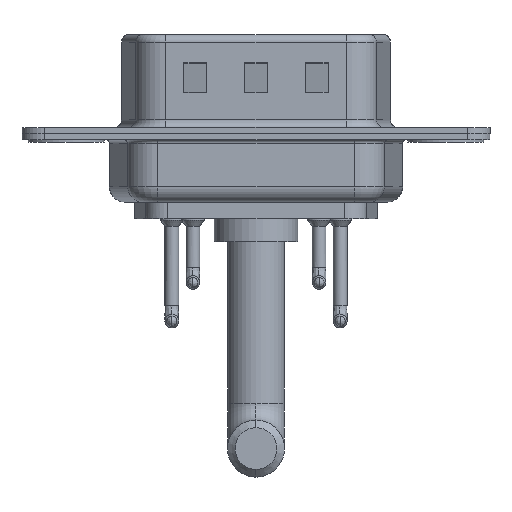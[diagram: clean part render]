
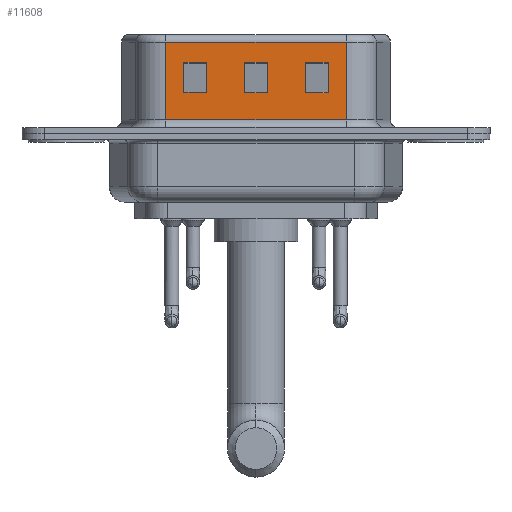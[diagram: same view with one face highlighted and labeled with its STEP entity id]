
A CAD part, front view. The second image highlights one B-rep face of the part: STEP entity #11608.
In plain terms, the highlighted planar face has unit normal (0, -1, 0).
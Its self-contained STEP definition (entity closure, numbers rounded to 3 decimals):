
#83 = ORIENTED_EDGE ( 'NONE', *, *, #14806, .T. ) ;
#181 = FACE_BOUND ( 'NONE', #15882, .T. ) ;
#237 = VECTOR ( 'NONE', #14333, 1000. ) ;
#532 = FACE_BOUND ( 'NONE', #3598, .T. ) ;
#615 = VERTEX_POINT ( 'NONE', #9459 ) ;
#1077 = CARTESIAN_POINT ( 'NONE',  ( 13.25, -4.55, 6.52 ) ) ;
#1397 = VERTEX_POINT ( 'NONE', #10139 ) ;
#1428 = AXIS2_PLACEMENT_3D ( 'NONE', #8686, #1691, #15089 ) ;
#1483 = CARTESIAN_POINT ( 'NONE',  ( 14.451, -4.55, 2.705 ) ) ;
#1499 = VERTEX_POINT ( 'NONE', #5333 ) ;
#1521 = VECTOR ( 'NONE', #3390, 1000. ) ;
#1559 = EDGE_CURVE ( 'NONE', #11625, #6355, #14482, .T. ) ;
#1678 = LINE ( 'NONE', #13912, #11077 ) ;
#1691 = DIRECTION ( 'NONE',  ( 0., 1., 0. ) ) ;
#1824 = CARTESIAN_POINT ( 'NONE',  ( 18.451, -4.55, 4.705 ) ) ;
#1938 = ORIENTED_EDGE ( 'NONE', *, *, #15453, .T. ) ;
#1942 = DIRECTION ( 'NONE',  ( -1., 0., 0. ) ) ;
#1975 = CARTESIAN_POINT ( 'NONE',  ( 6.549, -4.55, 6.52 ) ) ;
#2081 = VECTOR ( 'NONE', #13162, 1000. ) ;
#2189 = EDGE_CURVE ( 'NONE', #9253, #6253, #11804, .T. ) ;
#2249 = VECTOR ( 'NONE', #6692, 1000. ) ;
#2424 = CARTESIAN_POINT ( 'NONE',  ( 11.75, -4.55, 4.705 ) ) ;
#2632 = ORIENTED_EDGE ( 'NONE', *, *, #8674, .T. ) ;
#2973 = LINE ( 'NONE', #10772, #2249 ) ;
#3008 = VERTEX_POINT ( 'NONE', #13233 ) ;
#3295 = VERTEX_POINT ( 'NONE', #16240 ) ;
#3337 = VECTOR ( 'NONE', #1942, 1000. ) ;
#3390 = DIRECTION ( 'NONE',  ( 0., 0., -1. ) ) ;
#3515 = ORIENTED_EDGE ( 'NONE', *, *, #15458, .F. ) ;
#3539 = CARTESIAN_POINT ( 'NONE',  ( 9.25, -4.55, 4.705 ) ) ;
#3598 = EDGE_LOOP ( 'NONE', ( #4522, #8901, #6543, #4065 ) ) ;
#3662 = CARTESIAN_POINT ( 'NONE',  ( 18.451, -4.55, 6.52 ) ) ;
#3929 = CARTESIAN_POINT ( 'NONE',  ( 7.75, -4.55, 2.705 ) ) ;
#4065 = ORIENTED_EDGE ( 'NONE', *, *, #13582, .T. ) ;
#4439 = CARTESIAN_POINT ( 'NONE',  ( 22.451, -4.55, 2.705 ) ) ;
#4522 = ORIENTED_EDGE ( 'NONE', *, *, #8133, .T. ) ;
#4809 = LINE ( 'NONE', #17150, #2081 ) ;
#5047 = CARTESIAN_POINT ( 'NONE',  ( 9.25, -4.55, 6.52 ) ) ;
#5164 = DIRECTION ( 'NONE',  ( 0., 0., -1. ) ) ;
#5209 = CARTESIAN_POINT ( 'NONE',  ( 11.75, -4.55, 6.52 ) ) ;
#5333 = CARTESIAN_POINT ( 'NONE',  ( 18.451, -4.55, 6.02 ) ) ;
#5508 = VERTEX_POINT ( 'NONE', #3929 ) ;
#5896 = VECTOR ( 'NONE', #10975, 1000. ) ;
#5914 = VERTEX_POINT ( 'NONE', #17548 ) ;
#5937 = CARTESIAN_POINT ( 'NONE',  ( 13.25, -4.55, 4.705 ) ) ;
#6004 = VECTOR ( 'NONE', #11893, 1000. ) ;
#6127 = LINE ( 'NONE', #6396, #9691 ) ;
#6253 = VERTEX_POINT ( 'NONE', #14792 ) ;
#6355 = VERTEX_POINT ( 'NONE', #16469 ) ;
#6396 = CARTESIAN_POINT ( 'NONE',  ( 17.25, -4.55, 6.52 ) ) ;
#6412 = LINE ( 'NONE', #3662, #1521 ) ;
#6524 = CARTESIAN_POINT ( 'NONE',  ( 17.25, -4.55, 4.705 ) ) ;
#6543 = ORIENTED_EDGE ( 'NONE', *, *, #7555, .T. ) ;
#6565 = EDGE_CURVE ( 'NONE', #1499, #6721, #7399, .T. ) ;
#6692 = DIRECTION ( 'NONE',  ( 1., 0., 0. ) ) ;
#6703 = ORIENTED_EDGE ( 'NONE', *, *, #13167, .T. ) ;
#6721 = VERTEX_POINT ( 'NONE', #9350 ) ;
#6882 = DIRECTION ( 'NONE',  ( -1., 0., 0. ) ) ;
#7019 = VERTEX_POINT ( 'NONE', #2424 ) ;
#7227 = EDGE_CURVE ( 'NONE', #5914, #14096, #10193, .T. ) ;
#7256 = VERTEX_POINT ( 'NONE', #12682 ) ;
#7288 = DIRECTION ( 'NONE',  ( 0., 0., -1. ) ) ;
#7331 = VECTOR ( 'NONE', #7288, 1000. ) ;
#7399 = LINE ( 'NONE', #10510, #237 ) ;
#7555 = EDGE_CURVE ( 'NONE', #6355, #3295, #9478, .T. ) ;
#8004 = VECTOR ( 'NONE', #17128, 1000. ) ;
#8125 = ORIENTED_EDGE ( 'NONE', *, *, #2189, .T. ) ;
#8133 = EDGE_CURVE ( 'NONE', #7019, #11625, #8554, .T. ) ;
#8242 = FACE_BOUND ( 'NONE', #9436, .T. ) ;
#8493 = CARTESIAN_POINT ( 'NONE',  ( 15.75, -4.55, 2.705 ) ) ;
#8554 = LINE ( 'NONE', #1824, #14702 ) ;
#8674 = EDGE_CURVE ( 'NONE', #7256, #11106, #2973, .T. ) ;
#8686 = CARTESIAN_POINT ( 'NONE',  ( 18.451, -4.55, 6.52 ) ) ;
#8777 = EDGE_CURVE ( 'NONE', #6721, #3008, #12455, .T. ) ;
#8780 = ORIENTED_EDGE ( 'NONE', *, *, #12948, .T. ) ;
#8901 = ORIENTED_EDGE ( 'NONE', *, *, #1559, .T. ) ;
#8970 = DIRECTION ( 'NONE',  ( 0., 0., 1. ) ) ;
#9056 = CARTESIAN_POINT ( 'NONE',  ( 7.75, -4.55, 6.52 ) ) ;
#9253 = VERTEX_POINT ( 'NONE', #3539 ) ;
#9350 = CARTESIAN_POINT ( 'NONE',  ( 6.549, -4.55, 6.02 ) ) ;
#9371 = LINE ( 'NONE', #5209, #15043 ) ;
#9436 = EDGE_LOOP ( 'NONE', ( #8125, #83, #16252, #10934 ) ) ;
#9459 = CARTESIAN_POINT ( 'NONE',  ( 7.75, -4.55, 4.705 ) ) ;
#9478 = LINE ( 'NONE', #14890, #5896 ) ;
#9691 = VECTOR ( 'NONE', #14459, 1000. ) ;
#9886 = VECTOR ( 'NONE', #5164, 1000. ) ;
#10139 = CARTESIAN_POINT ( 'NONE',  ( 18.451, -4.55, 0.9 ) ) ;
#10168 = EDGE_LOOP ( 'NONE', ( #3515, #13315, #12248, #1938 ) ) ;
#10193 = LINE ( 'NONE', #4439, #3337 ) ;
#10510 = CARTESIAN_POINT ( 'NONE',  ( 18.451, -4.55, 6.02 ) ) ;
#10631 = DIRECTION ( 'NONE',  ( 0., 0., 1. ) ) ;
#10772 = CARTESIAN_POINT ( 'NONE',  ( 22.451, -4.55, 4.705 ) ) ;
#10934 = ORIENTED_EDGE ( 'NONE', *, *, #14036, .T. ) ;
#10975 = DIRECTION ( 'NONE',  ( -1., 0., 0. ) ) ;
#11077 = VECTOR ( 'NONE', #13569, 1000. ) ;
#11088 = FACE_OUTER_BOUND ( 'NONE', #10168, .T. ) ;
#11106 = VERTEX_POINT ( 'NONE', #6524 ) ;
#11608 = ADVANCED_FACE ( 'NONE', ( #8242, #181, #532, #11088 ), #14095, .F. ) ;
#11625 = VERTEX_POINT ( 'NONE', #5937 ) ;
#11804 = LINE ( 'NONE', #5047, #8004 ) ;
#11893 = DIRECTION ( 'NONE',  ( 0., 0., 1. ) ) ;
#12248 = ORIENTED_EDGE ( 'NONE', *, *, #8777, .T. ) ;
#12455 = LINE ( 'NONE', #1975, #7331 ) ;
#12562 = DIRECTION ( 'NONE',  ( 1., 0., 0. ) ) ;
#12682 = CARTESIAN_POINT ( 'NONE',  ( 15.75, -4.55, 4.705 ) ) ;
#12893 = LINE ( 'NONE', #9056, #16191 ) ;
#12948 = EDGE_CURVE ( 'NONE', #11106, #5914, #6127, .T. ) ;
#13162 = DIRECTION ( 'NONE',  ( 1., 0., 0. ) ) ;
#13167 = EDGE_CURVE ( 'NONE', #14096, #7256, #13495, .T. ) ;
#13233 = CARTESIAN_POINT ( 'NONE',  ( 6.549, -4.55, 0.9 ) ) ;
#13315 = ORIENTED_EDGE ( 'NONE', *, *, #6565, .T. ) ;
#13495 = LINE ( 'NONE', #17399, #6004 ) ;
#13569 = DIRECTION ( 'NONE',  ( 1., 0., 0. ) ) ;
#13582 = EDGE_CURVE ( 'NONE', #3295, #7019, #9371, .T. ) ;
#13632 = LINE ( 'NONE', #1483, #14514 ) ;
#13912 = CARTESIAN_POINT ( 'NONE',  ( 14.451, -4.55, 4.705 ) ) ;
#14036 = EDGE_CURVE ( 'NONE', #615, #9253, #1678, .T. ) ;
#14095 = PLANE ( 'NONE',  #1428 ) ;
#14096 = VERTEX_POINT ( 'NONE', #8493 ) ;
#14223 = EDGE_CURVE ( 'NONE', #5508, #615, #12893, .T. ) ;
#14333 = DIRECTION ( 'NONE',  ( -1., 0., 0. ) ) ;
#14437 = ORIENTED_EDGE ( 'NONE', *, *, #7227, .T. ) ;
#14459 = DIRECTION ( 'NONE',  ( 0., 0., -1. ) ) ;
#14482 = LINE ( 'NONE', #1077, #9886 ) ;
#14514 = VECTOR ( 'NONE', #6882, 1000. ) ;
#14702 = VECTOR ( 'NONE', #12562, 1000. ) ;
#14792 = CARTESIAN_POINT ( 'NONE',  ( 9.25, -4.55, 2.705 ) ) ;
#14806 = EDGE_CURVE ( 'NONE', #6253, #5508, #13632, .T. ) ;
#14890 = CARTESIAN_POINT ( 'NONE',  ( 18.451, -4.55, 2.705 ) ) ;
#15043 = VECTOR ( 'NONE', #10631, 1000. ) ;
#15089 = DIRECTION ( 'NONE',  ( -1., 0., 0. ) ) ;
#15453 = EDGE_CURVE ( 'NONE', #3008, #1397, #4809, .T. ) ;
#15458 = EDGE_CURVE ( 'NONE', #1499, #1397, #6412, .T. ) ;
#15882 = EDGE_LOOP ( 'NONE', ( #8780, #14437, #6703, #2632 ) ) ;
#16191 = VECTOR ( 'NONE', #8970, 1000. ) ;
#16240 = CARTESIAN_POINT ( 'NONE',  ( 11.75, -4.55, 2.705 ) ) ;
#16252 = ORIENTED_EDGE ( 'NONE', *, *, #14223, .T. ) ;
#16469 = CARTESIAN_POINT ( 'NONE',  ( 13.25, -4.55, 2.705 ) ) ;
#17128 = DIRECTION ( 'NONE',  ( 0., 0., -1. ) ) ;
#17150 = CARTESIAN_POINT ( 'NONE',  ( 18.451, -4.55, 0.9 ) ) ;
#17399 = CARTESIAN_POINT ( 'NONE',  ( 15.75, -4.55, 6.52 ) ) ;
#17548 = CARTESIAN_POINT ( 'NONE',  ( 17.25, -4.55, 2.705 ) ) ;
